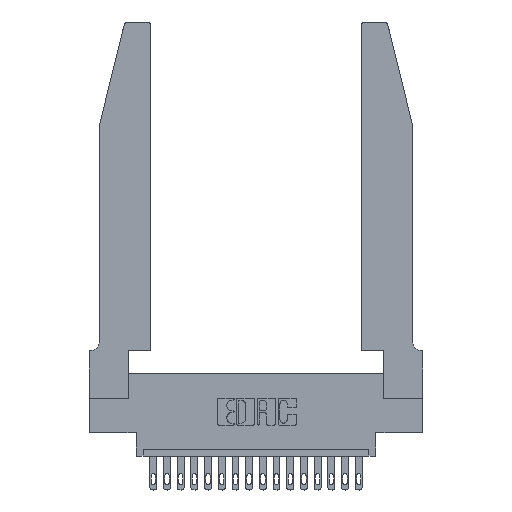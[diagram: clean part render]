
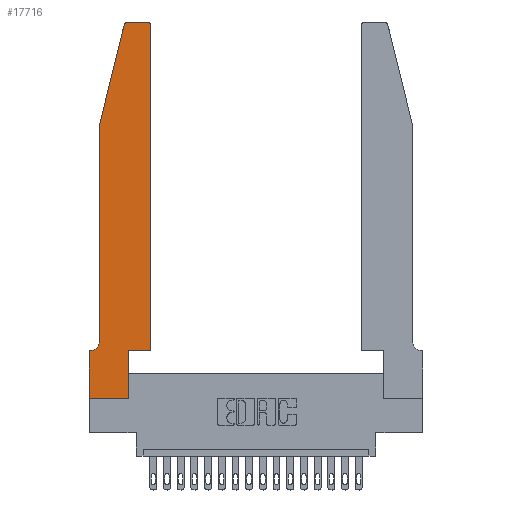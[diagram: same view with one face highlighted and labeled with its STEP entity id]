
A CAD part, top view. The second image highlights one B-rep face of the part: STEP entity #17716.
In plain terms, the highlighted planar face has unit normal (0, 0, 1).
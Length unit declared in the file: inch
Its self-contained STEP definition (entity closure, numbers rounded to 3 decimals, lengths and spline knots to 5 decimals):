
#127 = EDGE_CURVE ( 'NONE', #7648, #12777, #16721, .T. ) ;
#588 = DIRECTION ( 'NONE',  ( 0., 0., 1. ) ) ;
#837 = VECTOR ( 'NONE', #3070, 39.37008 ) ;
#872 = DIRECTION ( 'NONE',  ( 1., 0., 0. ) ) ;
#1073 = CARTESIAN_POINT ( 'NONE',  ( 0.284, 2.75, 0.37 ) ) ;
#1090 = LINE ( 'NONE', #5741, #13106 ) ;
#1111 = ORIENTED_EDGE ( 'NONE', *, *, #14739, .T. ) ;
#1128 = VECTOR ( 'NONE', #10461, 39.37008 ) ;
#1331 = CARTESIAN_POINT ( 'NONE',  ( 0.284, 2.72, 0.37 ) ) ;
#1611 = LINE ( 'NONE', #16962, #1128 ) ;
#1833 = CARTESIAN_POINT ( 'NONE',  ( 0.4505, 2.72, 0.37 ) ) ;
#1901 = CARTESIAN_POINT ( 'NONE',  ( 0.0055, 0.42, 0.37 ) ) ;
#1935 = VERTEX_POINT ( 'NONE', #15920 ) ;
#2342 = VERTEX_POINT ( 'NONE', #17533 ) ;
#2437 = CARTESIAN_POINT ( 'NONE',  ( 0.2865, 0.35, 0.37 ) ) ;
#2731 = CIRCLE ( 'NONE', #3019, 0.03 ) ;
#3019 = AXIS2_PLACEMENT_3D ( 'NONE', #14646, #588, #5201 ) ;
#3070 = DIRECTION ( 'NONE',  ( -0.239, -0.971, 0. ) ) ;
#3286 = DIRECTION ( 'NONE',  ( 1., 0., 0. ) ) ;
#3303 = CARTESIAN_POINT ( 'NONE',  ( 0.2605, 2.75, 0.37 ) ) ;
#3454 = DIRECTION ( 'NONE',  ( -1., 0., 0. ) ) ;
#3699 = CARTESIAN_POINT ( 'NONE',  ( 0.2865, 0.35, 0.37 ) ) ;
#3963 = EDGE_CURVE ( 'NONE', #17292, #19273, #16615, .T. ) ;
#4449 = AXIS2_PLACEMENT_3D ( 'NONE', #1331, #14293, #3286 ) ;
#4533 = CARTESIAN_POINT ( 'NONE',  ( 0.2865, 0., 0.37 ) ) ;
#4698 = LINE ( 'NONE', #9486, #7891 ) ;
#4720 = CARTESIAN_POINT ( 'NONE',  ( 0.0755, 2., 0.37 ) ) ;
#4826 = VERTEX_POINT ( 'NONE', #18652 ) ;
#4842 = EDGE_CURVE ( 'NONE', #19273, #6104, #16811, .T. ) ;
#5037 = CARTESIAN_POINT ( 'NONE',  ( 0.4505, 0.35, 0.37 ) ) ;
#5201 = DIRECTION ( 'NONE',  ( 1., 0., 0. ) ) ;
#5329 = PLANE ( 'NONE',  #10408 ) ;
#5390 = VECTOR ( 'NONE', #19564, 39.37008 ) ;
#5741 = CARTESIAN_POINT ( 'NONE',  ( 0.0755, 2., 0.37 ) ) ;
#5743 = LINE ( 'NONE', #7406, #19831 ) ;
#5833 = CARTESIAN_POINT ( 'NONE',  ( 0.25487, 2.72718, 0.37 ) ) ;
#6068 = VECTOR ( 'NONE', #18492, 39.37008 ) ;
#6104 = VERTEX_POINT ( 'NONE', #4720 ) ;
#6257 = CARTESIAN_POINT ( 'NONE',  ( 0.4205, 2.75, 0.37 ) ) ;
#7006 = LINE ( 'NONE', #5037, #19135 ) ;
#7267 = CIRCLE ( 'NONE', #8509, 0.07 ) ;
#7300 = CARTESIAN_POINT ( 'NONE',  ( 0., 0., 0.37 ) ) ;
#7406 = CARTESIAN_POINT ( 'NONE',  ( 0.4505, 0.35, 0.37 ) ) ;
#7648 = VERTEX_POINT ( 'NONE', #4533 ) ;
#7891 = VECTOR ( 'NONE', #18846, 39.37008 ) ;
#7991 = DIRECTION ( 'NONE',  ( 0., 0., -1. ) ) ;
#8187 = VERTEX_POINT ( 'NONE', #8478 ) ;
#8304 = VECTOR ( 'NONE', #10428, 39.37008 ) ;
#8478 = CARTESIAN_POINT ( 'NONE',  ( 0., 0., 0.37 ) ) ;
#8493 = CARTESIAN_POINT ( 'NONE',  ( 0., 0.35, 0.37 ) ) ;
#8509 = AXIS2_PLACEMENT_3D ( 'NONE', #1901, #7991, #3454 ) ;
#8701 = DIRECTION ( 'NONE',  ( 0., 0., 1. ) ) ;
#8820 = EDGE_CURVE ( 'NONE', #12777, #1935, #7006, .T. ) ;
#8934 = EDGE_CURVE ( 'NONE', #4826, #2342, #7267, .T. ) ;
#9465 = EDGE_CURVE ( 'NONE', #1935, #17080, #5743, .T. ) ;
#9486 = CARTESIAN_POINT ( 'NONE',  ( 0., 0., 0.37 ) ) ;
#9624 = EDGE_CURVE ( 'NONE', #2342, #16565, #1611, .T. ) ;
#9984 = ORIENTED_EDGE ( 'NONE', *, *, #4842, .T. ) ;
#10268 = ORIENTED_EDGE ( 'NONE', *, *, #18761, .T. ) ;
#10408 = AXIS2_PLACEMENT_3D ( 'NONE', #8493, #8701, #15054 ) ;
#10428 = DIRECTION ( 'NONE',  ( 0., 1., 0. ) ) ;
#10461 = DIRECTION ( 'NONE',  ( -1., 0., 0. ) ) ;
#10992 = ORIENTED_EDGE ( 'NONE', *, *, #13050, .T. ) ;
#11243 = ORIENTED_EDGE ( 'NONE', *, *, #3963, .T. ) ;
#11944 = DIRECTION ( 'NONE',  ( 0., -1., 0. ) ) ;
#11958 = DIRECTION ( 'NONE',  ( 0., 1., 0. ) ) ;
#12469 = ORIENTED_EDGE ( 'NONE', *, *, #9624, .T. ) ;
#12636 = FACE_OUTER_BOUND ( 'NONE', #17743, .T. ) ;
#12777 = VERTEX_POINT ( 'NONE', #2437 ) ;
#13050 = EDGE_CURVE ( 'NONE', #13181, #17292, #16500, .T. ) ;
#13106 = VECTOR ( 'NONE', #11944, 39.37008 ) ;
#13181 = VERTEX_POINT ( 'NONE', #6257 ) ;
#13456 = ORIENTED_EDGE ( 'NONE', *, *, #8934, .T. ) ;
#14064 = ORIENTED_EDGE ( 'NONE', *, *, #14805, .T. ) ;
#14293 = DIRECTION ( 'NONE',  ( 0., 0., 1. ) ) ;
#14646 = CARTESIAN_POINT ( 'NONE',  ( 0.4205, 2.72, 0.37 ) ) ;
#14739 = EDGE_CURVE ( 'NONE', #17080, #13181, #2731, .T. ) ;
#14805 = EDGE_CURVE ( 'NONE', #6104, #4826, #1090, .T. ) ;
#15054 = DIRECTION ( 'NONE',  ( 1., 0., 0. ) ) ;
#15083 = ORIENTED_EDGE ( 'NONE', *, *, #9465, .T. ) ;
#15541 = EDGE_CURVE ( 'NONE', #16565, #8187, #16431, .T. ) ;
#15920 = CARTESIAN_POINT ( 'NONE',  ( 0.4505, 0.35, 0.37 ) ) ;
#16431 = LINE ( 'NONE', #7300, #6068 ) ;
#16500 = LINE ( 'NONE', #3303, #5390 ) ;
#16565 = VERTEX_POINT ( 'NONE', #17121 ) ;
#16615 = CIRCLE ( 'NONE', #4449, 0.03 ) ;
#16721 = LINE ( 'NONE', #3699, #8304 ) ;
#16811 = LINE ( 'NONE', #16984, #837 ) ;
#16962 = CARTESIAN_POINT ( 'NONE',  ( 0.0755, 0.35, 0.37 ) ) ;
#16984 = CARTESIAN_POINT ( 'NONE',  ( 0.0755, 2., 0.37 ) ) ;
#17080 = VERTEX_POINT ( 'NONE', #1833 ) ;
#17121 = CARTESIAN_POINT ( 'NONE',  ( 0., 0.35, 0.37 ) ) ;
#17292 = VERTEX_POINT ( 'NONE', #1073 ) ;
#17307 = ORIENTED_EDGE ( 'NONE', *, *, #8820, .T. ) ;
#17533 = CARTESIAN_POINT ( 'NONE',  ( 0.0055, 0.35, 0.37 ) ) ;
#17716 = ADVANCED_FACE ( 'NONE', ( #12636 ), #5329, .T. ) ;
#17743 = EDGE_LOOP ( 'NONE', ( #10992, #11243, #9984, #14064, #13456, #12469, #19548, #10268, #19784, #17307, #15083, #1111 ) ) ;
#18492 = DIRECTION ( 'NONE',  ( 0., -1., 0. ) ) ;
#18652 = CARTESIAN_POINT ( 'NONE',  ( 0.0755, 0.42, 0.37 ) ) ;
#18761 = EDGE_CURVE ( 'NONE', #8187, #7648, #4698, .T. ) ;
#18846 = DIRECTION ( 'NONE',  ( 1., 0., 0. ) ) ;
#19135 = VECTOR ( 'NONE', #872, 39.37008 ) ;
#19273 = VERTEX_POINT ( 'NONE', #5833 ) ;
#19548 = ORIENTED_EDGE ( 'NONE', *, *, #15541, .T. ) ;
#19564 = DIRECTION ( 'NONE',  ( -1., 0., 0. ) ) ;
#19784 = ORIENTED_EDGE ( 'NONE', *, *, #127, .T. ) ;
#19831 = VECTOR ( 'NONE', #11958, 39.37008 ) ;
